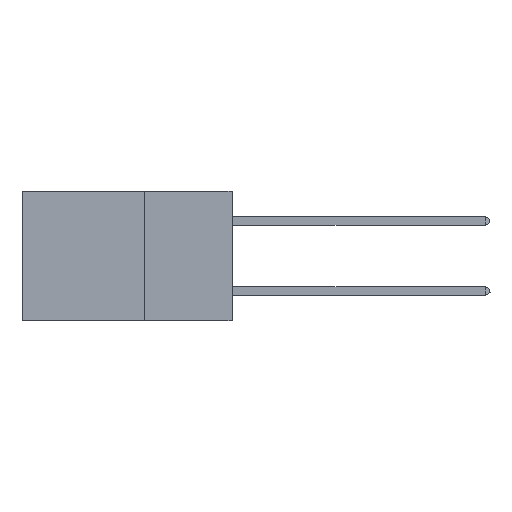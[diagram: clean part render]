
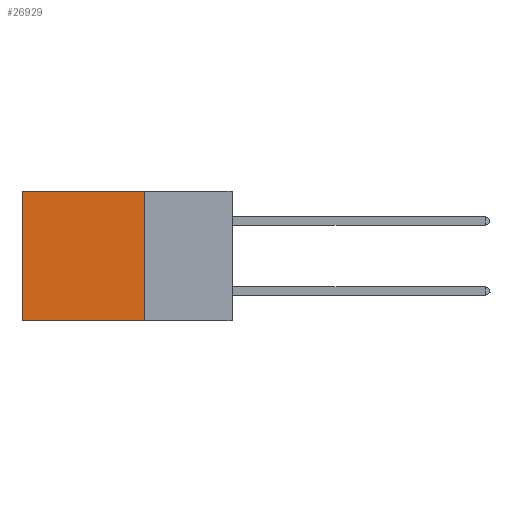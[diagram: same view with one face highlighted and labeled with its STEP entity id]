
A CAD part, left-side view. The second image highlights one B-rep face of the part: STEP entity #26929.
In plain terms, the highlighted planar face has unit normal (-1, 0, 0).
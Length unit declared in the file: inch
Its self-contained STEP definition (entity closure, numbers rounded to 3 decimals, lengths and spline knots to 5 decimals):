
#99 = CARTESIAN_POINT ( 'NONE',  ( 0.2875, 0.25, -0.37 ) ) ;
#1227 = VECTOR ( 'NONE', #6213, 39.37008 ) ;
#2002 = PLANE ( 'NONE',  #8550 ) ;
#2899 = ORIENTED_EDGE ( 'NONE', *, *, #27765, .T. ) ;
#3439 = CARTESIAN_POINT ( 'NONE',  ( 0.2875, 0.25, 0. ) ) ;
#3789 = VERTEX_POINT ( 'NONE', #9469 ) ;
#3938 = EDGE_CURVE ( 'NONE', #3789, #32738, #15903, .T. ) ;
#4653 = DIRECTION ( 'NONE',  ( 0., 0., -1. ) ) ;
#4911 = DIRECTION ( 'NONE',  ( 0., 0., -1. ) ) ;
#6213 = DIRECTION ( 'NONE',  ( 0., 1., 0. ) ) ;
#7455 = DIRECTION ( 'NONE',  ( 1., 0., 0. ) ) ;
#8028 = EDGE_LOOP ( 'NONE', ( #2899, #15293, #26015, #31695 ) ) ;
#8122 = CARTESIAN_POINT ( 'NONE',  ( 0.2875, 0.6, 0. ) ) ;
#8550 = AXIS2_PLACEMENT_3D ( 'NONE', #22109, #7455, #4911 ) ;
#9317 = VECTOR ( 'NONE', #26456, 39.37008 ) ;
#9469 = CARTESIAN_POINT ( 'NONE',  ( 0.2875, 0.25, -0.37 ) ) ;
#9609 = VECTOR ( 'NONE', #17294, 39.37008 ) ;
#11167 = EDGE_CURVE ( 'NONE', #32768, #32424, #12961, .T. ) ;
#12239 = CARTESIAN_POINT ( 'NONE',  ( 0.2875, 0.6, -0.37 ) ) ;
#12961 = LINE ( 'NONE', #23036, #1227 ) ;
#15293 = ORIENTED_EDGE ( 'NONE', *, *, #3938, .F. ) ;
#15903 = LINE ( 'NONE', #99, #9609 ) ;
#17294 = DIRECTION ( 'NONE',  ( 0., 1., 0. ) ) ;
#18573 = EDGE_CURVE ( 'NONE', #32768, #3789, #37224, .T. ) ;
#20962 = CARTESIAN_POINT ( 'NONE',  ( 0.2875, 0.6, 0. ) ) ;
#22109 = CARTESIAN_POINT ( 'NONE',  ( 0.2875, 0.25, 0. ) ) ;
#23036 = CARTESIAN_POINT ( 'NONE',  ( 0.2875, 0.25, 0. ) ) ;
#26015 = ORIENTED_EDGE ( 'NONE', *, *, #18573, .F. ) ;
#26456 = DIRECTION ( 'NONE',  ( 0., 0., -1. ) ) ;
#26829 = CARTESIAN_POINT ( 'NONE',  ( 0.2875, 0.25, 0. ) ) ;
#26929 = ADVANCED_FACE ( 'NONE', ( #35814 ), #2002, .F. ) ;
#27765 = EDGE_CURVE ( 'NONE', #32424, #32738, #32126, .T. ) ;
#31695 = ORIENTED_EDGE ( 'NONE', *, *, #11167, .T. ) ;
#32126 = LINE ( 'NONE', #20962, #34339 ) ;
#32424 = VERTEX_POINT ( 'NONE', #8122 ) ;
#32738 = VERTEX_POINT ( 'NONE', #12239 ) ;
#32768 = VERTEX_POINT ( 'NONE', #26829 ) ;
#34339 = VECTOR ( 'NONE', #4653, 39.37008 ) ;
#35814 = FACE_OUTER_BOUND ( 'NONE', #8028, .T. ) ;
#37224 = LINE ( 'NONE', #3439, #9317 ) ;
